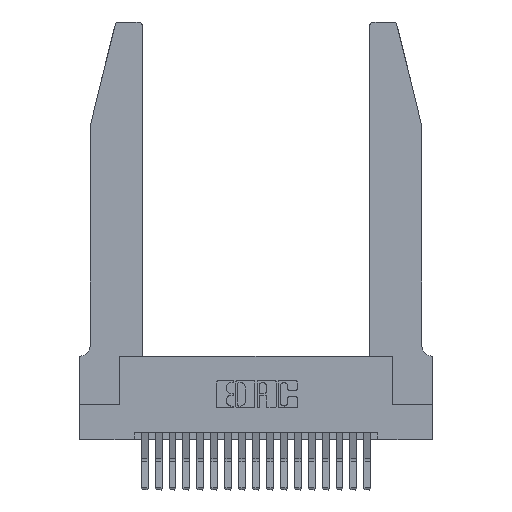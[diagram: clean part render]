
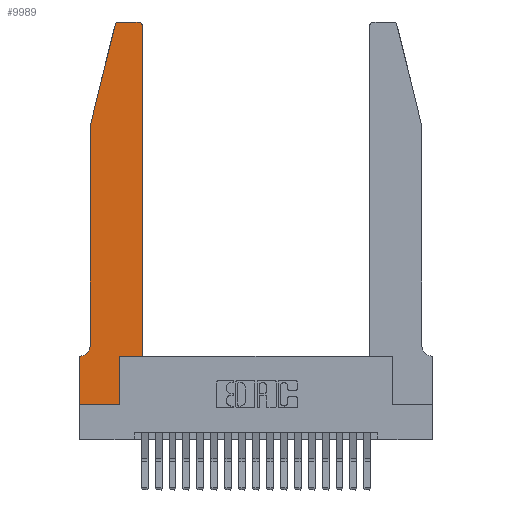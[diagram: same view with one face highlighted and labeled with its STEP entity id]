
A CAD part, top view. The second image highlights one B-rep face of the part: STEP entity #9989.
In plain terms, the highlighted planar face has unit normal (0, 0, 1).
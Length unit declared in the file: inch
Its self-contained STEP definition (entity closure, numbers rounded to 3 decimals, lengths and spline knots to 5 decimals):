
#213 = CARTESIAN_POINT ( 'NONE',  ( 0.0755, 2., 0.37 ) ) ;
#313 = CIRCLE ( 'NONE', #3715, 0.03 ) ;
#822 = CARTESIAN_POINT ( 'NONE',  ( 0., 0., 0.37 ) ) ;
#1189 = ORIENTED_EDGE ( 'NONE', *, *, #1744, .T. ) ;
#1315 = VECTOR ( 'NONE', #8448, 39.37008 ) ;
#1428 = EDGE_CURVE ( 'NONE', #6403, #3399, #12283, .T. ) ;
#1713 = DIRECTION ( 'NONE',  ( -1., 0., 0. ) ) ;
#1744 = EDGE_CURVE ( 'NONE', #3751, #9732, #19814, .T. ) ;
#1951 = CARTESIAN_POINT ( 'NONE',  ( 0.284, 2.75, 0.37 ) ) ;
#1952 = EDGE_CURVE ( 'NONE', #4881, #4836, #7062, .T. ) ;
#1974 = AXIS2_PLACEMENT_3D ( 'NONE', #6757, #15059, #16750 ) ;
#2461 = VERTEX_POINT ( 'NONE', #1951 ) ;
#2768 = CARTESIAN_POINT ( 'NONE',  ( 0.2605, 2.75, 0.37 ) ) ;
#2980 = ORIENTED_EDGE ( 'NONE', *, *, #1428, .T. ) ;
#3007 = EDGE_CURVE ( 'NONE', #4836, #17738, #16251, .T. ) ;
#3267 = VECTOR ( 'NONE', #15993, 39.37008 ) ;
#3399 = VERTEX_POINT ( 'NONE', #12555 ) ;
#3405 = VECTOR ( 'NONE', #14643, 39.37008 ) ;
#3715 = AXIS2_PLACEMENT_3D ( 'NONE', #17696, #7749, #11101 ) ;
#3751 = VERTEX_POINT ( 'NONE', #8837 ) ;
#3912 = ORIENTED_EDGE ( 'NONE', *, *, #6147, .T. ) ;
#3954 = CARTESIAN_POINT ( 'NONE',  ( 0., 0.35, 0.37 ) ) ;
#4126 = VERTEX_POINT ( 'NONE', #14606 ) ;
#4294 = ORIENTED_EDGE ( 'NONE', *, *, #3007, .T. ) ;
#4386 = LINE ( 'NONE', #5668, #8310 ) ;
#4468 = VECTOR ( 'NONE', #14473, 39.37008 ) ;
#4637 = ORIENTED_EDGE ( 'NONE', *, *, #16683, .T. ) ;
#4652 = ORIENTED_EDGE ( 'NONE', *, *, #1952, .T. ) ;
#4836 = VERTEX_POINT ( 'NONE', #20160 ) ;
#4869 = VECTOR ( 'NONE', #11876, 39.37008 ) ;
#4881 = VERTEX_POINT ( 'NONE', #213 ) ;
#4963 = CARTESIAN_POINT ( 'NONE',  ( 0.0755, 2., 0.37 ) ) ;
#5242 = CARTESIAN_POINT ( 'NONE',  ( 0.4205, 2.75, 0.37 ) ) ;
#5549 = DIRECTION ( 'NONE',  ( 1., 0., 0. ) ) ;
#5668 = CARTESIAN_POINT ( 'NONE',  ( 0., 0., 0.37 ) ) ;
#5965 = ORIENTED_EDGE ( 'NONE', *, *, #6441, .T. ) ;
#6147 = EDGE_CURVE ( 'NONE', #14426, #6403, #4386, .T. ) ;
#6218 = CARTESIAN_POINT ( 'NONE',  ( 0., 0.35, 0.37 ) ) ;
#6403 = VERTEX_POINT ( 'NONE', #11564 ) ;
#6441 = EDGE_CURVE ( 'NONE', #17738, #9073, #8801, .T. ) ;
#6755 = AXIS2_PLACEMENT_3D ( 'NONE', #8341, #8483, #16724 ) ;
#6757 = CARTESIAN_POINT ( 'NONE',  ( 0.0055, 0.42, 0.37 ) ) ;
#7053 = CARTESIAN_POINT ( 'NONE',  ( 0.0755, 2., 0.37 ) ) ;
#7062 = LINE ( 'NONE', #4963, #3405 ) ;
#7299 = VECTOR ( 'NONE', #17800, 39.37008 ) ;
#7749 = DIRECTION ( 'NONE',  ( 0., 0., 1. ) ) ;
#7833 = ORIENTED_EDGE ( 'NONE', *, *, #18210, .T. ) ;
#8310 = VECTOR ( 'NONE', #20586, 39.37008 ) ;
#8341 = CARTESIAN_POINT ( 'NONE',  ( 0.284, 2.72, 0.37 ) ) ;
#8448 = DIRECTION ( 'NONE',  ( 0., 1., 0. ) ) ;
#8483 = DIRECTION ( 'NONE',  ( 0., 0., 1. ) ) ;
#8801 = LINE ( 'NONE', #21505, #15319 ) ;
#8808 = CARTESIAN_POINT ( 'NONE',  ( 0., 0., 0.37 ) ) ;
#8837 = CARTESIAN_POINT ( 'NONE',  ( 0.4505, 0.35, 0.37 ) ) ;
#9073 = VERTEX_POINT ( 'NONE', #6218 ) ;
#9732 = VERTEX_POINT ( 'NONE', #18186 ) ;
#9785 = LINE ( 'NONE', #822, #3267 ) ;
#9989 = ADVANCED_FACE ( 'NONE', ( #19073 ), #12048, .T. ) ;
#10111 = LINE ( 'NONE', #12301, #4869 ) ;
#10957 = DIRECTION ( 'NONE',  ( -1., 0., 0. ) ) ;
#11101 = DIRECTION ( 'NONE',  ( 1., 0., 0. ) ) ;
#11219 = ORIENTED_EDGE ( 'NONE', *, *, #12857, .T. ) ;
#11564 = CARTESIAN_POINT ( 'NONE',  ( 0.2865, 0., 0.37 ) ) ;
#11876 = DIRECTION ( 'NONE',  ( 1., 0., 0. ) ) ;
#12048 = PLANE ( 'NONE',  #18915 ) ;
#12283 = LINE ( 'NONE', #20951, #4468 ) ;
#12301 = CARTESIAN_POINT ( 'NONE',  ( 0.4505, 0.35, 0.37 ) ) ;
#12555 = CARTESIAN_POINT ( 'NONE',  ( 0.2865, 0.35, 0.37 ) ) ;
#12734 = EDGE_LOOP ( 'NONE', ( #16786, #4637, #11219, #4652, #4294, #5965, #7833, #3912, #2980, #20307, #1189, #16592 ) ) ;
#12857 = EDGE_CURVE ( 'NONE', #4126, #4881, #19471, .T. ) ;
#14295 = EDGE_CURVE ( 'NONE', #3399, #3751, #10111, .T. ) ;
#14334 = VERTEX_POINT ( 'NONE', #5242 ) ;
#14426 = VERTEX_POINT ( 'NONE', #8808 ) ;
#14473 = DIRECTION ( 'NONE',  ( 0., 1., 0. ) ) ;
#14606 = CARTESIAN_POINT ( 'NONE',  ( 0.25487, 2.72718, 0.37 ) ) ;
#14643 = DIRECTION ( 'NONE',  ( 0., -1., 0. ) ) ;
#14747 = CIRCLE ( 'NONE', #6755, 0.03 ) ;
#14961 = VECTOR ( 'NONE', #10957, 39.37008 ) ;
#15059 = DIRECTION ( 'NONE',  ( 0., 0., -1. ) ) ;
#15208 = CARTESIAN_POINT ( 'NONE',  ( 0.4505, 0.35, 0.37 ) ) ;
#15317 = DIRECTION ( 'NONE',  ( 0., 0., 1. ) ) ;
#15319 = VECTOR ( 'NONE', #1713, 39.37008 ) ;
#15993 = DIRECTION ( 'NONE',  ( 0., -1., 0. ) ) ;
#16251 = CIRCLE ( 'NONE', #1974, 0.07 ) ;
#16592 = ORIENTED_EDGE ( 'NONE', *, *, #19889, .T. ) ;
#16683 = EDGE_CURVE ( 'NONE', #2461, #4126, #14747, .T. ) ;
#16724 = DIRECTION ( 'NONE',  ( 1., 0., 0. ) ) ;
#16750 = DIRECTION ( 'NONE',  ( -1., 0., 0. ) ) ;
#16786 = ORIENTED_EDGE ( 'NONE', *, *, #18885, .T. ) ;
#17696 = CARTESIAN_POINT ( 'NONE',  ( 0.4205, 2.72, 0.37 ) ) ;
#17738 = VERTEX_POINT ( 'NONE', #18013 ) ;
#17800 = DIRECTION ( 'NONE',  ( -0.239, -0.971, 0. ) ) ;
#18013 = CARTESIAN_POINT ( 'NONE',  ( 0.0055, 0.35, 0.37 ) ) ;
#18186 = CARTESIAN_POINT ( 'NONE',  ( 0.4505, 2.72, 0.37 ) ) ;
#18210 = EDGE_CURVE ( 'NONE', #9073, #14426, #9785, .T. ) ;
#18885 = EDGE_CURVE ( 'NONE', #14334, #2461, #20165, .T. ) ;
#18915 = AXIS2_PLACEMENT_3D ( 'NONE', #3954, #15317, #5549 ) ;
#19073 = FACE_OUTER_BOUND ( 'NONE', #12734, .T. ) ;
#19471 = LINE ( 'NONE', #7053, #7299 ) ;
#19814 = LINE ( 'NONE', #15208, #1315 ) ;
#19889 = EDGE_CURVE ( 'NONE', #9732, #14334, #313, .T. ) ;
#20160 = CARTESIAN_POINT ( 'NONE',  ( 0.0755, 0.42, 0.37 ) ) ;
#20165 = LINE ( 'NONE', #2768, #14961 ) ;
#20307 = ORIENTED_EDGE ( 'NONE', *, *, #14295, .T. ) ;
#20586 = DIRECTION ( 'NONE',  ( 1., 0., 0. ) ) ;
#20951 = CARTESIAN_POINT ( 'NONE',  ( 0.2865, 0.35, 0.37 ) ) ;
#21505 = CARTESIAN_POINT ( 'NONE',  ( 0.0755, 0.35, 0.37 ) ) ;
